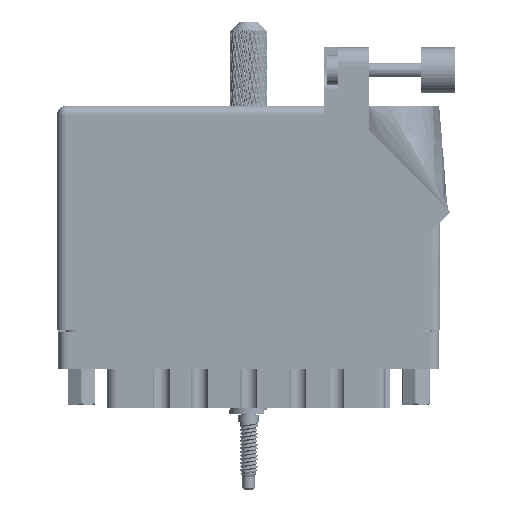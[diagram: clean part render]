
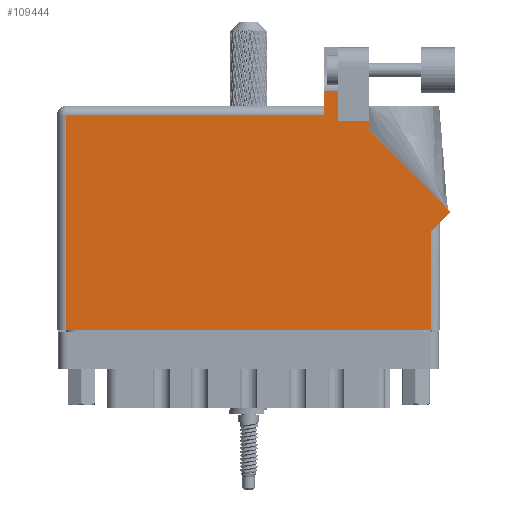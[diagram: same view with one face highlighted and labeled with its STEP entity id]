
A CAD part, front view. The second image highlights one B-rep face of the part: STEP entity #109444.
In plain terms, the highlighted face is planar.
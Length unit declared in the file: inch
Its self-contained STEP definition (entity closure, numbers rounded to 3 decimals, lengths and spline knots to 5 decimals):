
#1596 = PLANE ( 'NONE',  #111383 ) ;
#2080 = VECTOR ( 'NONE', #52115, 39.37008 ) ;
#2843 = VERTEX_POINT ( 'NONE', #51393 ) ;
#3094 = CARTESIAN_POINT ( 'NONE',  ( 2.612, 0.737, 0. ) ) ;
#3891 = VECTOR ( 'NONE', #119167, 39.37008 ) ;
#4647 = CARTESIAN_POINT ( 'NONE',  ( 1.913, 1.6315, 0. ) ) ;
#5511 = EDGE_CURVE ( 'NONE', #125797, #8437, #50140, .T. ) ;
#5523 = VECTOR ( 'NONE', #82199, 39.37008 ) ;
#8437 = VERTEX_POINT ( 'NONE', #124194 ) ;
#8521 = VERTEX_POINT ( 'NONE', #44907 ) ;
#9616 = CARTESIAN_POINT ( 'NONE',  ( 2.24377, 1.6315, 0. ) ) ;
#9632 = VERTEX_POINT ( 'NONE', #4647 ) ;
#10362 = VECTOR ( 'NONE', #52190, 39.37008 ) ;
#12555 = CARTESIAN_POINT ( 'NONE',  ( 2.126, 1.43, 0. ) ) ;
#13016 = ORIENTED_EDGE ( 'NONE', *, *, #5511, .T. ) ;
#15360 = DIRECTION ( 'NONE',  ( 0., 1., 0. ) ) ;
#15417 = VERTEX_POINT ( 'NONE', #72384 ) ;
#15636 = LINE ( 'NONE', #77980, #59032 ) ;
#15868 = CARTESIAN_POINT ( 'NONE',  ( 1.819, 1.468, 0. ) ) ;
#16218 = CARTESIAN_POINT ( 'NONE',  ( 0.062, 1.468, 0. ) ) ;
#16696 = EDGE_CURVE ( 'NONE', #8521, #9632, #62435, .T. ) ;
#17100 = CARTESIAN_POINT ( 'NONE',  ( 0., 0., 0. ) ) ;
#18388 = ORIENTED_EDGE ( 'NONE', *, *, #62536, .T. ) ;
#23799 = VERTEX_POINT ( 'NONE', #15868 ) ;
#24057 = ORIENTED_EDGE ( 'NONE', *, *, #67073, .T. ) ;
#25055 = CARTESIAN_POINT ( 'NONE',  ( 0., 1.468, 0. ) ) ;
#26693 = VECTOR ( 'NONE', #41830, 39.37008 ) ;
#29834 = CARTESIAN_POINT ( 'NONE',  ( 2.126, 1.43, 0. ) ) ;
#30172 = VERTEX_POINT ( 'NONE', #66034 ) ;
#30928 = EDGE_CURVE ( 'NONE', #23799, #125699, #53341, .T. ) ;
#32279 = CARTESIAN_POINT ( 'NONE',  ( 2.55, 0.675, 0. ) ) ;
#32833 = LINE ( 'NONE', #74835, #65206 ) ;
#33440 = ORIENTED_EDGE ( 'NONE', *, *, #113608, .T. ) ;
#37859 = EDGE_CURVE ( 'NONE', #125699, #125797, #87563, .T. ) ;
#40338 = CARTESIAN_POINT ( 'NONE',  ( 2.126, 1.36442, 0. ) ) ;
#40880 = VECTOR ( 'NONE', #65432, 39.37008 ) ;
#41830 = DIRECTION ( 'NONE',  ( 0., 1., 0. ) ) ;
#44115 = EDGE_CURVE ( 'NONE', #9632, #2843, #121347, .T. ) ;
#44866 = EDGE_CURVE ( 'NONE', #15417, #117708, #118135, .T. ) ;
#44907 = CARTESIAN_POINT ( 'NONE',  ( 1.913, 1.43, 0. ) ) ;
#47611 = EDGE_LOOP ( 'NONE', ( #113194, #115603, #97092, #107928, #104968, #13016, #18388, #68364, #24057, #123688, #33440 ) ) ;
#50140 = LINE ( 'NONE', #17100, #126148 ) ;
#51393 = CARTESIAN_POINT ( 'NONE',  ( 1.819, 1.6315, 0. ) ) ;
#52115 = DIRECTION ( 'NONE',  ( 0., -1., 0. ) ) ;
#52190 = DIRECTION ( 'NONE',  ( 0.707, 0.707, 0. ) ) ;
#53341 = LINE ( 'NONE', #25055, #40880 ) ;
#57997 = DIRECTION ( 'NONE',  ( 0., -1., 0. ) ) ;
#59032 = VECTOR ( 'NONE', #57997, 39.37008 ) ;
#61813 = CARTESIAN_POINT ( 'NONE',  ( 2.68271, 0.80771, 0. ) ) ;
#62435 = LINE ( 'NONE', #71745, #26693 ) ;
#62536 = EDGE_CURVE ( 'NONE', #8437, #63805, #32833, .T. ) ;
#63805 = VERTEX_POINT ( 'NONE', #32279 ) ;
#65206 = VECTOR ( 'NONE', #15360, 39.37008 ) ;
#65432 = DIRECTION ( 'NONE',  ( -1., 0., 0. ) ) ;
#66034 = CARTESIAN_POINT ( 'NONE',  ( 2.68271, 0.80771, 0. ) ) ;
#67073 = EDGE_CURVE ( 'NONE', #30172, #15417, #69167, .T. ) ;
#68364 = ORIENTED_EDGE ( 'NONE', *, *, #73330, .T. ) ;
#69167 = LINE ( 'NONE', #61813, #5523 ) ;
#69961 = CARTESIAN_POINT ( 'NONE',  ( 0.062, 0., 0. ) ) ;
#70700 = DIRECTION ( 'NONE',  ( 0., 1., 0. ) ) ;
#71465 = FACE_OUTER_BOUND ( 'NONE', #47611, .T. ) ;
#71745 = CARTESIAN_POINT ( 'NONE',  ( 1.913, 1.43, 0. ) ) ;
#72384 = CARTESIAN_POINT ( 'NONE',  ( 2.126, 1.36442, 0. ) ) ;
#73330 = EDGE_CURVE ( 'NONE', #63805, #30172, #100379, .T. ) ;
#74835 = CARTESIAN_POINT ( 'NONE',  ( 2.55, 0.737, 0. ) ) ;
#77412 = DIRECTION ( 'NONE',  ( 1., 0., 0. ) ) ;
#77980 = CARTESIAN_POINT ( 'NONE',  ( 1.819, 1.53, 0. ) ) ;
#80492 = DIRECTION ( 'NONE',  ( -1., 0., 0. ) ) ;
#81476 = DIRECTION ( 'NONE',  ( -1., 0., 0. ) ) ;
#82199 = DIRECTION ( 'NONE',  ( -0.707, 0.707, 0. ) ) ;
#85768 = VECTOR ( 'NONE', #80492, 39.37008 ) ;
#87563 = LINE ( 'NONE', #118866, #2080 ) ;
#89343 = LINE ( 'NONE', #29834, #3891 ) ;
#90305 = VECTOR ( 'NONE', #70700, 39.37008 ) ;
#92607 = EDGE_CURVE ( 'NONE', #2843, #23799, #15636, .T. ) ;
#97092 = ORIENTED_EDGE ( 'NONE', *, *, #92607, .T. ) ;
#100379 = LINE ( 'NONE', #3094, #10362 ) ;
#104968 = ORIENTED_EDGE ( 'NONE', *, *, #37859, .T. ) ;
#107928 = ORIENTED_EDGE ( 'NONE', *, *, #30928, .T. ) ;
#109444 = ADVANCED_FACE ( 'NONE', ( #71465 ), #1596, .F. ) ;
#109599 = CARTESIAN_POINT ( 'NONE',  ( 0., 1.53, 0. ) ) ;
#111383 = AXIS2_PLACEMENT_3D ( 'NONE', #109599, #122183, #81476 ) ;
#113194 = ORIENTED_EDGE ( 'NONE', *, *, #16696, .T. ) ;
#113608 = EDGE_CURVE ( 'NONE', #117708, #8521, #89343, .T. ) ;
#115603 = ORIENTED_EDGE ( 'NONE', *, *, #44115, .T. ) ;
#117708 = VERTEX_POINT ( 'NONE', #12555 ) ;
#118135 = LINE ( 'NONE', #40338, #90305 ) ;
#118866 = CARTESIAN_POINT ( 'NONE',  ( 0.062, 0., 0. ) ) ;
#119167 = DIRECTION ( 'NONE',  ( -1., 0., 0. ) ) ;
#121347 = LINE ( 'NONE', #9616, #85768 ) ;
#122183 = DIRECTION ( 'NONE',  ( 0., 0., -1. ) ) ;
#123688 = ORIENTED_EDGE ( 'NONE', *, *, #44866, .T. ) ;
#124194 = CARTESIAN_POINT ( 'NONE',  ( 2.55, 0., 0. ) ) ;
#125699 = VERTEX_POINT ( 'NONE', #16218 ) ;
#125797 = VERTEX_POINT ( 'NONE', #69961 ) ;
#126148 = VECTOR ( 'NONE', #77412, 39.37008 ) ;
